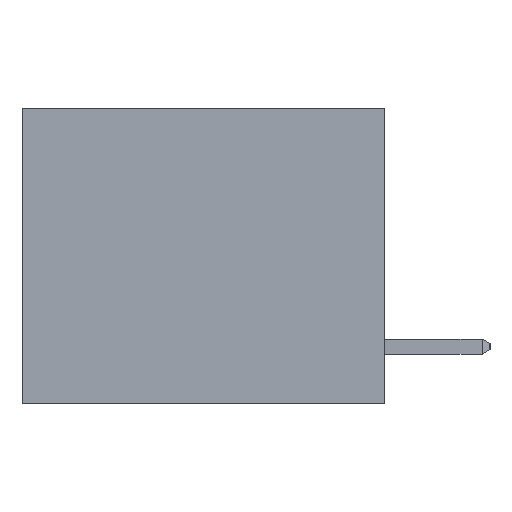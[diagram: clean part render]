
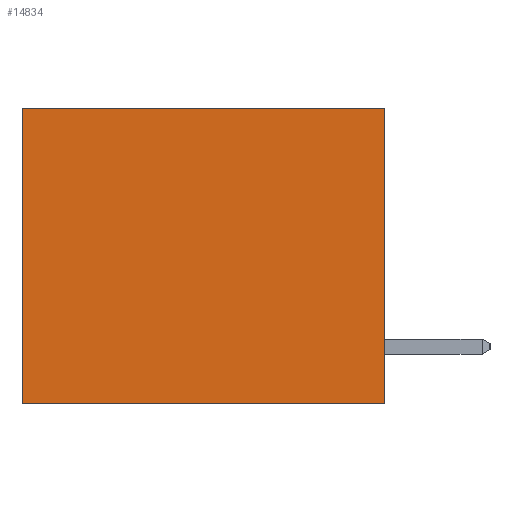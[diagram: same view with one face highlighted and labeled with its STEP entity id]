
A CAD part, left-side view. The second image highlights one B-rep face of the part: STEP entity #14834.
In plain terms, the highlighted planar face has unit normal (-1, 0, 0).
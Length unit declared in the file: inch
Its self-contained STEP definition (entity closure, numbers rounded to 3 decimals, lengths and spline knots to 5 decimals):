
#2600 = DIRECTION ( 'NONE',  ( 0., 1., 0. ) ) ;
#3204 = ORIENTED_EDGE ( 'NONE', *, *, #3763, .F. ) ;
#3685 = DIRECTION ( 'NONE',  ( 0., 0., -1. ) ) ;
#3763 = EDGE_CURVE ( 'NONE', #10239, #22965, #20559, .T. ) ;
#4137 = ORIENTED_EDGE ( 'NONE', *, *, #11643, .T. ) ;
#4324 = VECTOR ( 'NONE', #15094, 39.37008 ) ;
#4696 = VERTEX_POINT ( 'NONE', #21405 ) ;
#5802 = CARTESIAN_POINT ( 'NONE',  ( 0.3165, 0., -0.49 ) ) ;
#5877 = CARTESIAN_POINT ( 'NONE',  ( 0.3165, 0.6, -0.49 ) ) ;
#5983 = CARTESIAN_POINT ( 'NONE',  ( 0.3165, 0., -0.49 ) ) ;
#7899 = PLANE ( 'NONE',  #27859 ) ;
#10239 = VERTEX_POINT ( 'NONE', #23376 ) ;
#10973 = ORIENTED_EDGE ( 'NONE', *, *, #16336, .T. ) ;
#11304 = VERTEX_POINT ( 'NONE', #28595 ) ;
#11643 = EDGE_CURVE ( 'NONE', #11304, #22965, #16339, .T. ) ;
#13611 = VECTOR ( 'NONE', #2600, 39.37008 ) ;
#14834 = ADVANCED_FACE ( 'NONE', ( #24608 ), #7899, .F. ) ;
#15094 = DIRECTION ( 'NONE',  ( 0., 0., -1. ) ) ;
#15131 = CARTESIAN_POINT ( 'NONE',  ( 0.3165, 0., -0.49 ) ) ;
#15206 = DIRECTION ( 'NONE',  ( 0., 1., 0. ) ) ;
#15727 = LINE ( 'NONE', #25072, #13611 ) ;
#16336 = EDGE_CURVE ( 'NONE', #4696, #11304, #15727, .T. ) ;
#16339 = LINE ( 'NONE', #5877, #4324 ) ;
#17624 = EDGE_CURVE ( 'NONE', #4696, #10239, #22372, .T. ) ;
#20559 = LINE ( 'NONE', #5983, #22302 ) ;
#21405 = CARTESIAN_POINT ( 'NONE',  ( 0.3165, 0., 0. ) ) ;
#21530 = DIRECTION ( 'NONE',  ( 1., 0., 0. ) ) ;
#21650 = EDGE_LOOP ( 'NONE', ( #4137, #3204, #24046, #10973 ) ) ;
#22302 = VECTOR ( 'NONE', #15206, 39.37008 ) ;
#22372 = LINE ( 'NONE', #15131, #26596 ) ;
#22965 = VERTEX_POINT ( 'NONE', #26261 ) ;
#23376 = CARTESIAN_POINT ( 'NONE',  ( 0.3165, 0., -0.49 ) ) ;
#23795 = DIRECTION ( 'NONE',  ( 0., 0., -1. ) ) ;
#24046 = ORIENTED_EDGE ( 'NONE', *, *, #17624, .F. ) ;
#24608 = FACE_OUTER_BOUND ( 'NONE', #21650, .T. ) ;
#25072 = CARTESIAN_POINT ( 'NONE',  ( 0.3165, 0., 0. ) ) ;
#26261 = CARTESIAN_POINT ( 'NONE',  ( 0.3165, 0.6, -0.49 ) ) ;
#26596 = VECTOR ( 'NONE', #3685, 39.37008 ) ;
#27859 = AXIS2_PLACEMENT_3D ( 'NONE', #5802, #21530, #23795 ) ;
#28595 = CARTESIAN_POINT ( 'NONE',  ( 0.3165, 0.6, 0. ) ) ;
